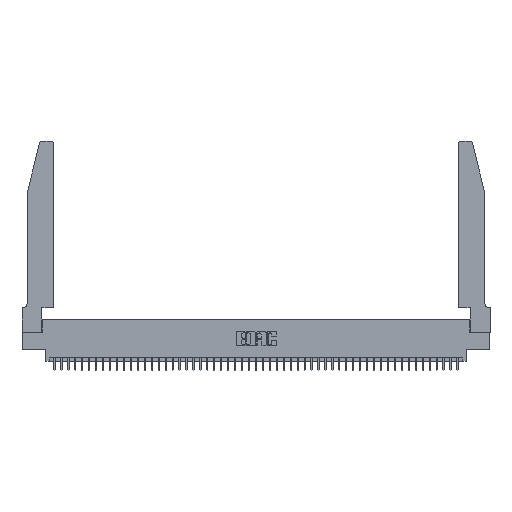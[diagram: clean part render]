
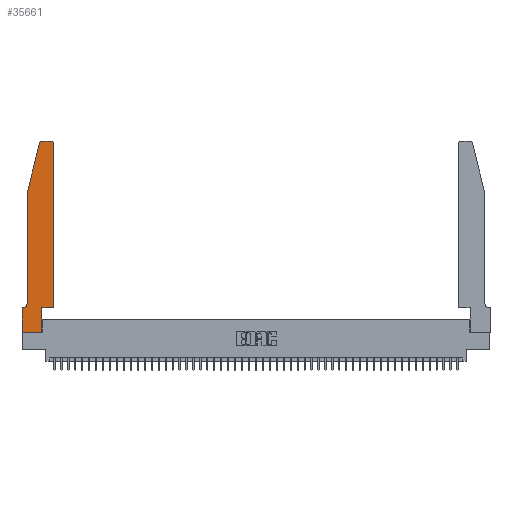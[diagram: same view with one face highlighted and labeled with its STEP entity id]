
A CAD part, top view. The second image highlights one B-rep face of the part: STEP entity #35661.
In plain terms, the highlighted planar face has unit normal (0, 0, 1).
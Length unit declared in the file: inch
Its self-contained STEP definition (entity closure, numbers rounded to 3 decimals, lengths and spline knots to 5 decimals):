
#1 = DIRECTION ( 'NONE',  ( 0., 0., 1. ) ) ;
#1115 = VERTEX_POINT ( 'NONE', #41308 ) ;
#1320 = VECTOR ( 'NONE', #13805, 39.37008 ) ;
#1485 = CARTESIAN_POINT ( 'NONE',  ( 0., 0., 0.37 ) ) ;
#2266 = ORIENTED_EDGE ( 'NONE', *, *, #32436, .T. ) ;
#2489 = VECTOR ( 'NONE', #13309, 39.37008 ) ;
#2500 = DIRECTION ( 'NONE',  ( 0., 0., 1. ) ) ;
#2643 = VERTEX_POINT ( 'NONE', #15267 ) ;
#3094 = CIRCLE ( 'NONE', #47428, 0.03 ) ;
#4094 = CARTESIAN_POINT ( 'NONE',  ( 0.0055, 0.35, 0.37 ) ) ;
#4299 = LINE ( 'NONE', #34093, #44035 ) ;
#4776 = LINE ( 'NONE', #19924, #35568 ) ;
#5685 = CARTESIAN_POINT ( 'NONE',  ( 0.0755, 0.42, 0.37 ) ) ;
#6012 = VERTEX_POINT ( 'NONE', #42439 ) ;
#6783 = DIRECTION ( 'NONE',  ( -1., 0., 0. ) ) ;
#7858 = VERTEX_POINT ( 'NONE', #20551 ) ;
#8175 = CARTESIAN_POINT ( 'NONE',  ( 0.4505, 2.72, 0.37 ) ) ;
#9363 = DIRECTION ( 'NONE',  ( 0., 0., 1. ) ) ;
#10454 = LINE ( 'NONE', #32846, #18649 ) ;
#10503 = ORIENTED_EDGE ( 'NONE', *, *, #34620, .T. ) ;
#10704 = VERTEX_POINT ( 'NONE', #5685 ) ;
#10979 = VECTOR ( 'NONE', #46995, 39.37008 ) ;
#11467 = DIRECTION ( 'NONE',  ( 0., 0., -1. ) ) ;
#11582 = EDGE_CURVE ( 'NONE', #17645, #1115, #14516, .T. ) ;
#11873 = EDGE_CURVE ( 'NONE', #10704, #23066, #19878, .T. ) ;
#12910 = VERTEX_POINT ( 'NONE', #23416 ) ;
#13309 = DIRECTION ( 'NONE',  ( 1., 0., 0. ) ) ;
#13805 = DIRECTION ( 'NONE',  ( 0., 1., 0. ) ) ;
#14059 = DIRECTION ( 'NONE',  ( 1., 0., 0. ) ) ;
#14126 = CARTESIAN_POINT ( 'NONE',  ( 0.4205, 2.72, 0.37 ) ) ;
#14295 = CIRCLE ( 'NONE', #42065, 0.03 ) ;
#14516 = LINE ( 'NONE', #29681, #31050 ) ;
#15104 = DIRECTION ( 'NONE',  ( 1., 0., 0. ) ) ;
#15110 = ORIENTED_EDGE ( 'NONE', *, *, #18295, .T. ) ;
#15267 = CARTESIAN_POINT ( 'NONE',  ( 0.2865, 0.35, 0.37 ) ) ;
#15570 = ORIENTED_EDGE ( 'NONE', *, *, #11873, .T. ) ;
#15934 = DIRECTION ( 'NONE',  ( 1., 0., 0. ) ) ;
#17162 = VECTOR ( 'NONE', #30623, 39.37008 ) ;
#17592 = DIRECTION ( 'NONE',  ( 1., 0., 0. ) ) ;
#17645 = VERTEX_POINT ( 'NONE', #21016 ) ;
#18295 = EDGE_CURVE ( 'NONE', #2643, #7858, #4299, .T. ) ;
#18649 = VECTOR ( 'NONE', #47940, 39.37008 ) ;
#19115 = ORIENTED_EDGE ( 'NONE', *, *, #41515, .T. ) ;
#19830 = ORIENTED_EDGE ( 'NONE', *, *, #36789, .T. ) ;
#19878 = CIRCLE ( 'NONE', #20760, 0.07 ) ;
#19924 = CARTESIAN_POINT ( 'NONE',  ( 0.0755, 2., 0.37 ) ) ;
#20489 = CARTESIAN_POINT ( 'NONE',  ( 0.4205, 2.75, 0.37 ) ) ;
#20551 = CARTESIAN_POINT ( 'NONE',  ( 0.4505, 0.35, 0.37 ) ) ;
#20578 = EDGE_CURVE ( 'NONE', #47710, #2643, #48004, .T. ) ;
#20598 = VERTEX_POINT ( 'NONE', #20489 ) ;
#20760 = AXIS2_PLACEMENT_3D ( 'NONE', #37808, #11467, #6783 ) ;
#20848 = CARTESIAN_POINT ( 'NONE',  ( 0., 0.35, 0.37 ) ) ;
#21016 = CARTESIAN_POINT ( 'NONE',  ( 0., 0.35, 0.37 ) ) ;
#21796 = VECTOR ( 'NONE', #44382, 39.37008 ) ;
#22684 = LINE ( 'NONE', #34342, #17162 ) ;
#23066 = VERTEX_POINT ( 'NONE', #4094 ) ;
#23416 = CARTESIAN_POINT ( 'NONE',  ( 0.284, 2.75, 0.37 ) ) ;
#23823 = LINE ( 'NONE', #1485, #2489 ) ;
#23953 = ORIENTED_EDGE ( 'NONE', *, *, #45838, .T. ) ;
#24410 = DIRECTION ( 'NONE',  ( 0., -1., 0. ) ) ;
#25427 = EDGE_LOOP ( 'NONE', ( #10503, #34990, #19830, #44202, #15570, #30035, #28049, #23953, #47584, #15110, #2266, #19115 ) ) ;
#25498 = CARTESIAN_POINT ( 'NONE',  ( 0.2865, 0., 0.37 ) ) ;
#25865 = AXIS2_PLACEMENT_3D ( 'NONE', #20848, #2500, #17592 ) ;
#28049 = ORIENTED_EDGE ( 'NONE', *, *, #11582, .T. ) ;
#28257 = CARTESIAN_POINT ( 'NONE',  ( 0.284, 2.72, 0.37 ) ) ;
#29240 = LINE ( 'NONE', #40657, #1320 ) ;
#29270 = CARTESIAN_POINT ( 'NONE',  ( 0.2605, 2.75, 0.37 ) ) ;
#29681 = CARTESIAN_POINT ( 'NONE',  ( 0., 0., 0.37 ) ) ;
#30035 = ORIENTED_EDGE ( 'NONE', *, *, #31545, .T. ) ;
#30623 = DIRECTION ( 'NONE',  ( -0.239, -0.971, 0. ) ) ;
#31050 = VECTOR ( 'NONE', #44799, 39.37008 ) ;
#31545 = EDGE_CURVE ( 'NONE', #23066, #17645, #10454, .T. ) ;
#31783 = FACE_OUTER_BOUND ( 'NONE', #25427, .T. ) ;
#31905 = CARTESIAN_POINT ( 'NONE',  ( 0.2865, 0.35, 0.37 ) ) ;
#32436 = EDGE_CURVE ( 'NONE', #7858, #35598, #29240, .T. ) ;
#32846 = CARTESIAN_POINT ( 'NONE',  ( 0.0755, 0.35, 0.37 ) ) ;
#33908 = EDGE_CURVE ( 'NONE', #40303, #10704, #4776, .T. ) ;
#34093 = CARTESIAN_POINT ( 'NONE',  ( 0.4505, 0.35, 0.37 ) ) ;
#34342 = CARTESIAN_POINT ( 'NONE',  ( 0.0755, 2., 0.37 ) ) ;
#34620 = EDGE_CURVE ( 'NONE', #20598, #12910, #48108, .T. ) ;
#34990 = ORIENTED_EDGE ( 'NONE', *, *, #45882, .T. ) ;
#35568 = VECTOR ( 'NONE', #24410, 39.37008 ) ;
#35598 = VERTEX_POINT ( 'NONE', #8175 ) ;
#35661 = ADVANCED_FACE ( 'NONE', ( #31783 ), #46871, .T. ) ;
#36789 = EDGE_CURVE ( 'NONE', #6012, #40303, #22684, .T. ) ;
#37808 = CARTESIAN_POINT ( 'NONE',  ( 0.0055, 0.42, 0.37 ) ) ;
#40303 = VERTEX_POINT ( 'NONE', #40437 ) ;
#40437 = CARTESIAN_POINT ( 'NONE',  ( 0.0755, 2., 0.37 ) ) ;
#40657 = CARTESIAN_POINT ( 'NONE',  ( 0.4505, 0.35, 0.37 ) ) ;
#41308 = CARTESIAN_POINT ( 'NONE',  ( 0., 0., 0.37 ) ) ;
#41515 = EDGE_CURVE ( 'NONE', #35598, #20598, #3094, .T. ) ;
#42065 = AXIS2_PLACEMENT_3D ( 'NONE', #28257, #9363, #14059 ) ;
#42439 = CARTESIAN_POINT ( 'NONE',  ( 0.25487, 2.72718, 0.37 ) ) ;
#44035 = VECTOR ( 'NONE', #15934, 39.37008 ) ;
#44202 = ORIENTED_EDGE ( 'NONE', *, *, #33908, .T. ) ;
#44382 = DIRECTION ( 'NONE',  ( -1., 0., 0. ) ) ;
#44799 = DIRECTION ( 'NONE',  ( 0., -1., 0. ) ) ;
#45838 = EDGE_CURVE ( 'NONE', #1115, #47710, #23823, .T. ) ;
#45882 = EDGE_CURVE ( 'NONE', #12910, #6012, #14295, .T. ) ;
#46871 = PLANE ( 'NONE',  #25865 ) ;
#46995 = DIRECTION ( 'NONE',  ( 0., 1., 0. ) ) ;
#47428 = AXIS2_PLACEMENT_3D ( 'NONE', #14126, #1, #15104 ) ;
#47584 = ORIENTED_EDGE ( 'NONE', *, *, #20578, .T. ) ;
#47710 = VERTEX_POINT ( 'NONE', #25498 ) ;
#47940 = DIRECTION ( 'NONE',  ( -1., 0., 0. ) ) ;
#48004 = LINE ( 'NONE', #31905, #10979 ) ;
#48108 = LINE ( 'NONE', #29270, #21796 ) ;
